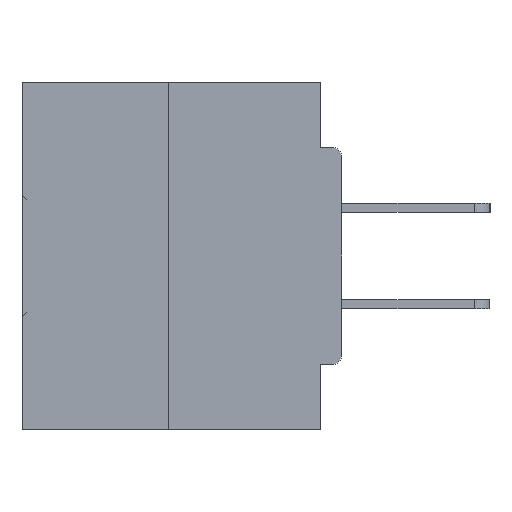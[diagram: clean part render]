
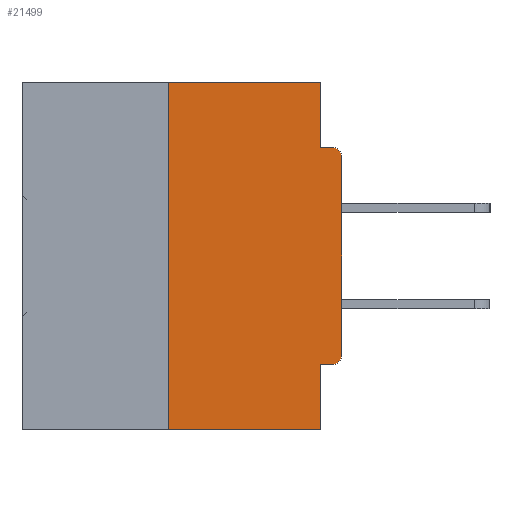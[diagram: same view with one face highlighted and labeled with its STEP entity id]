
A CAD part, left-side view. The second image highlights one B-rep face of the part: STEP entity #21499.
In plain terms, the highlighted planar face has unit normal (-1, 0, 0).
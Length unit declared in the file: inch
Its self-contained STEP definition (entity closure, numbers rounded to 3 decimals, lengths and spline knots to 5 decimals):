
#79 = LINE ( 'NONE', #25805, #31790 ) ;
#625 = VERTEX_POINT ( 'NONE', #37418 ) ;
#813 = AXIS2_PLACEMENT_3D ( 'NONE', #36866, #26797, #2180 ) ;
#1750 = ORIENTED_EDGE ( 'NONE', *, *, #32162, .F. ) ;
#2180 = DIRECTION ( 'NONE',  ( 0., 0., -1. ) ) ;
#6176 = VECTOR ( 'NONE', #34077, 39.37008 ) ;
#6205 = CARTESIAN_POINT ( 'NONE',  ( 0., 0.031, -0.5 ) ) ;
#7127 = VERTEX_POINT ( 'NONE', #24195 ) ;
#7228 = DIRECTION ( 'NONE',  ( 1., 0., 0. ) ) ;
#7669 = DIRECTION ( 'NONE',  ( 0., -1., 0. ) ) ;
#8701 = LINE ( 'NONE', #18017, #16911 ) ;
#8967 = EDGE_CURVE ( 'NONE', #625, #9795, #8701, .T. ) ;
#9795 = VERTEX_POINT ( 'NONE', #6205 ) ;
#10187 = PLANE ( 'NONE',  #29763 ) ;
#10325 = CIRCLE ( 'NONE', #41753, 0.015 ) ;
#10327 = LINE ( 'NONE', #44762, #40240 ) ;
#12181 = CARTESIAN_POINT ( 'NONE',  ( 0., 0., -0.3915 ) ) ;
#13080 = EDGE_CURVE ( 'NONE', #41190, #9795, #10327, .T. ) ;
#14216 = LINE ( 'NONE', #40321, #42582 ) ;
#14382 = LINE ( 'NONE', #39545, #6176 ) ;
#14666 = FACE_OUTER_BOUND ( 'NONE', #31733, .T. ) ;
#14850 = ORIENTED_EDGE ( 'NONE', *, *, #33532, .F. ) ;
#16907 = ORIENTED_EDGE ( 'NONE', *, *, #8967, .F. ) ;
#16911 = VECTOR ( 'NONE', #38779, 39.37008 ) ;
#17023 = VERTEX_POINT ( 'NONE', #18127 ) ;
#17468 = CARTESIAN_POINT ( 'NONE',  ( 0., 0.015, -0.4065 ) ) ;
#17605 = EDGE_CURVE ( 'NONE', #21425, #625, #34688, .T. ) ;
#17737 = LINE ( 'NONE', #20952, #44572 ) ;
#18017 = CARTESIAN_POINT ( 'NONE',  ( 0., 0.031, -0.5 ) ) ;
#18127 = CARTESIAN_POINT ( 'NONE',  ( 0., 0.015, -0.0935 ) ) ;
#18656 = CARTESIAN_POINT ( 'NONE',  ( 0., 0., -0.4065 ) ) ;
#18682 = ORIENTED_EDGE ( 'NONE', *, *, #36754, .F. ) ;
#18927 = VERTEX_POINT ( 'NONE', #37823 ) ;
#19412 = VECTOR ( 'NONE', #43092, 39.37008 ) ;
#20069 = ORIENTED_EDGE ( 'NONE', *, *, #17605, .F. ) ;
#20531 = EDGE_CURVE ( 'NONE', #18927, #17023, #10325, .T. ) ;
#20721 = ORIENTED_EDGE ( 'NONE', *, *, #31782, .F. ) ;
#20952 = CARTESIAN_POINT ( 'NONE',  ( 0., 0.46, 0. ) ) ;
#21275 = LINE ( 'NONE', #33309, #31054 ) ;
#21425 = VERTEX_POINT ( 'NONE', #17468 ) ;
#21499 = ADVANCED_FACE ( 'NONE', ( #14666 ), #10187, .F. ) ;
#23066 = ORIENTED_EDGE ( 'NONE', *, *, #13080, .T. ) ;
#23303 = VERTEX_POINT ( 'NONE', #44267 ) ;
#24164 = VERTEX_POINT ( 'NONE', #12181 ) ;
#24195 = CARTESIAN_POINT ( 'NONE',  ( 0., 0.031, 0. ) ) ;
#25805 = CARTESIAN_POINT ( 'NONE',  ( 0., 0.031, 0. ) ) ;
#25951 = CARTESIAN_POINT ( 'NONE',  ( 0., 0.25, -0.5 ) ) ;
#25988 = CARTESIAN_POINT ( 'NONE',  ( 0., 0.015, -0.1085 ) ) ;
#26554 = CARTESIAN_POINT ( 'NONE',  ( 0., 0.46, 0. ) ) ;
#26644 = ORIENTED_EDGE ( 'NONE', *, *, #44025, .T. ) ;
#26797 = DIRECTION ( 'NONE',  ( -1., 0., 0. ) ) ;
#29763 = AXIS2_PLACEMENT_3D ( 'NONE', #26554, #7228, #44668 ) ;
#30807 = DIRECTION ( 'NONE',  ( 0., 0., 1. ) ) ;
#31054 = VECTOR ( 'NONE', #32993, 39.37008 ) ;
#31733 = EDGE_LOOP ( 'NONE', ( #18682, #14850, #23066, #16907, #20069, #34592, #26644, #36465, #20721, #1750 ) ) ;
#31782 = EDGE_CURVE ( 'NONE', #32740, #17023, #14382, .T. ) ;
#31790 = VECTOR ( 'NONE', #39034, 39.37008 ) ;
#32162 = EDGE_CURVE ( 'NONE', #7127, #32740, #79, .T. ) ;
#32740 = VERTEX_POINT ( 'NONE', #42204 ) ;
#32984 = DIRECTION ( 'NONE',  ( 0., 0., -1. ) ) ;
#32993 = DIRECTION ( 'NONE',  ( 0., 0., 1. ) ) ;
#33309 = CARTESIAN_POINT ( 'NONE',  ( 0., 0., 0. ) ) ;
#33532 = EDGE_CURVE ( 'NONE', #41190, #23303, #14216, .T. ) ;
#34077 = DIRECTION ( 'NONE',  ( 0., -1., 0. ) ) ;
#34592 = ORIENTED_EDGE ( 'NONE', *, *, #34680, .T. ) ;
#34680 = EDGE_CURVE ( 'NONE', #21425, #24164, #34930, .T. ) ;
#34688 = LINE ( 'NONE', #18656, #19412 ) ;
#34930 = CIRCLE ( 'NONE', #813, 0.015 ) ;
#36221 = DIRECTION ( 'NONE',  ( -1., 0., 0. ) ) ;
#36465 = ORIENTED_EDGE ( 'NONE', *, *, #20531, .T. ) ;
#36754 = EDGE_CURVE ( 'NONE', #23303, #7127, #17737, .T. ) ;
#36866 = CARTESIAN_POINT ( 'NONE',  ( 0., 0.015, -0.3915 ) ) ;
#37418 = CARTESIAN_POINT ( 'NONE',  ( 0., 0.031, -0.4065 ) ) ;
#37823 = CARTESIAN_POINT ( 'NONE',  ( 0., 0., -0.1085 ) ) ;
#38779 = DIRECTION ( 'NONE',  ( 0., 0., -1. ) ) ;
#39034 = DIRECTION ( 'NONE',  ( 0., 0., -1. ) ) ;
#39545 = CARTESIAN_POINT ( 'NONE',  ( 0., 0., -0.0935 ) ) ;
#39851 = DIRECTION ( 'NONE',  ( 0., -1., 0. ) ) ;
#40240 = VECTOR ( 'NONE', #7669, 39.37008 ) ;
#40321 = CARTESIAN_POINT ( 'NONE',  ( 0., 0.25, 0. ) ) ;
#41190 = VERTEX_POINT ( 'NONE', #25951 ) ;
#41753 = AXIS2_PLACEMENT_3D ( 'NONE', #25988, #36221, #32984 ) ;
#42204 = CARTESIAN_POINT ( 'NONE',  ( 0., 0.031, -0.0935 ) ) ;
#42582 = VECTOR ( 'NONE', #30807, 39.37008 ) ;
#43092 = DIRECTION ( 'NONE',  ( 0., 1., 0. ) ) ;
#44025 = EDGE_CURVE ( 'NONE', #24164, #18927, #21275, .T. ) ;
#44267 = CARTESIAN_POINT ( 'NONE',  ( 0., 0.25, 0. ) ) ;
#44572 = VECTOR ( 'NONE', #39851, 39.37008 ) ;
#44668 = DIRECTION ( 'NONE',  ( 0., 0., -1. ) ) ;
#44762 = CARTESIAN_POINT ( 'NONE',  ( 0., 0.46, -0.5 ) ) ;
